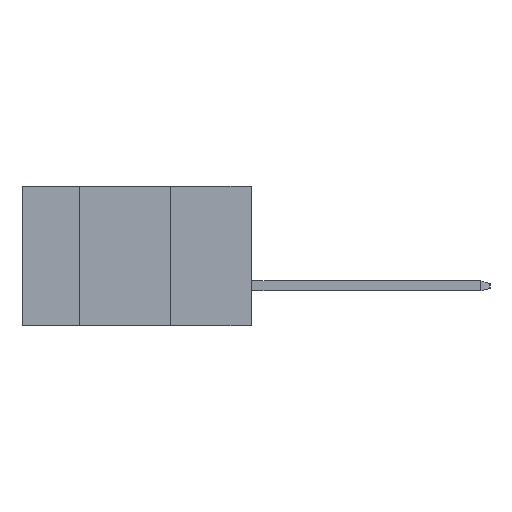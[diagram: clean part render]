
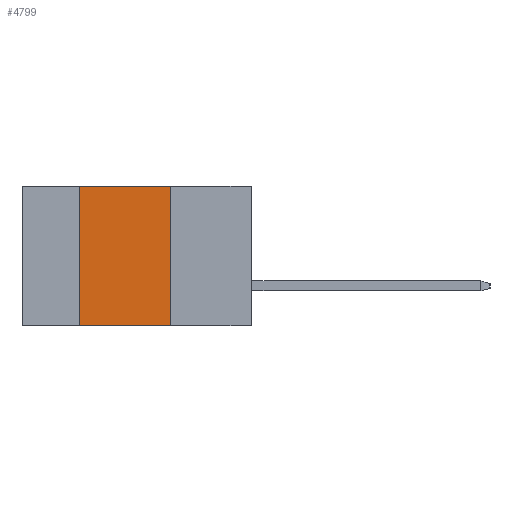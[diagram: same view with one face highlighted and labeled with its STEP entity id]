
A CAD part, left-side view. The second image highlights one B-rep face of the part: STEP entity #4799.
In plain terms, the highlighted planar face has unit normal (-1, 0, 0).
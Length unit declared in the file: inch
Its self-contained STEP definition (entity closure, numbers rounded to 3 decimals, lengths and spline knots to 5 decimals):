
#515 = FACE_OUTER_BOUND ( 'NONE', #2993, .T. ) ;
#604 = CARTESIAN_POINT ( 'NONE',  ( 0., 0.72, 0. ) ) ;
#661 = DIRECTION ( 'NONE',  ( 0., -1., 0. ) ) ;
#1434 = VERTEX_POINT ( 'NONE', #8236 ) ;
#1753 = EDGE_CURVE ( 'NONE', #5642, #1434, #2192, .T. ) ;
#1972 = VECTOR ( 'NONE', #10552, 39.37008 ) ;
#2184 = DIRECTION ( 'NONE',  ( 0., -1., 0. ) ) ;
#2192 = LINE ( 'NONE', #5873, #1972 ) ;
#2440 = ORIENTED_EDGE ( 'NONE', *, *, #9878, .T. ) ;
#2461 = PLANE ( 'NONE',  #5425 ) ;
#2671 = ORIENTED_EDGE ( 'NONE', *, *, #1753, .F. ) ;
#2975 = CARTESIAN_POINT ( 'NONE',  ( 0., 0.72, -0.437 ) ) ;
#2993 = EDGE_LOOP ( 'NONE', ( #2671, #5861, #3224, #2440 ) ) ;
#3224 = ORIENTED_EDGE ( 'NONE', *, *, #10604, .F. ) ;
#3308 = EDGE_CURVE ( 'NONE', #12030, #5642, #4385, .T. ) ;
#3343 = CARTESIAN_POINT ( 'NONE',  ( 0., 0.254, 0. ) ) ;
#3511 = DIRECTION ( 'NONE',  ( 0., 0., -1. ) ) ;
#3617 = VECTOR ( 'NONE', #4835, 39.37008 ) ;
#4244 = DIRECTION ( 'NONE',  ( 1., 0., 0. ) ) ;
#4385 = LINE ( 'NONE', #604, #10543 ) ;
#4799 = ADVANCED_FACE ( 'NONE', ( #515 ), #2461, .F. ) ;
#4835 = DIRECTION ( 'NONE',  ( 0., 0., 1. ) ) ;
#4903 = LINE ( 'NONE', #8487, #3617 ) ;
#5425 = AXIS2_PLACEMENT_3D ( 'NONE', #11800, #4244, #3511 ) ;
#5642 = VERTEX_POINT ( 'NONE', #3343 ) ;
#5861 = ORIENTED_EDGE ( 'NONE', *, *, #3308, .F. ) ;
#5873 = CARTESIAN_POINT ( 'NONE',  ( 0., 0.254, -0.437 ) ) ;
#7148 = VECTOR ( 'NONE', #2184, 39.37008 ) ;
#8236 = CARTESIAN_POINT ( 'NONE',  ( 0., 0.254, -0.437 ) ) ;
#8487 = CARTESIAN_POINT ( 'NONE',  ( 0., 0.54, -0.437 ) ) ;
#9878 = EDGE_CURVE ( 'NONE', #10382, #1434, #11389, .T. ) ;
#10333 = CARTESIAN_POINT ( 'NONE',  ( 0., 0.54, 0. ) ) ;
#10382 = VERTEX_POINT ( 'NONE', #11658 ) ;
#10543 = VECTOR ( 'NONE', #661, 39.37008 ) ;
#10552 = DIRECTION ( 'NONE',  ( 0., 0., -1. ) ) ;
#10604 = EDGE_CURVE ( 'NONE', #10382, #12030, #4903, .T. ) ;
#11389 = LINE ( 'NONE', #2975, #7148 ) ;
#11658 = CARTESIAN_POINT ( 'NONE',  ( 0., 0.54, -0.437 ) ) ;
#11800 = CARTESIAN_POINT ( 'NONE',  ( 0., 0.72, 0. ) ) ;
#12030 = VERTEX_POINT ( 'NONE', #10333 ) ;
